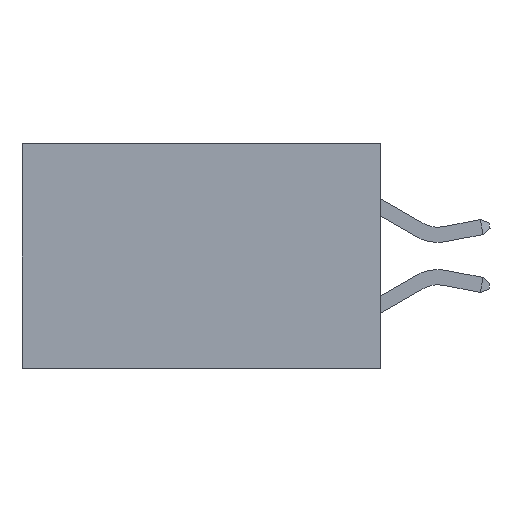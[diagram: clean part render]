
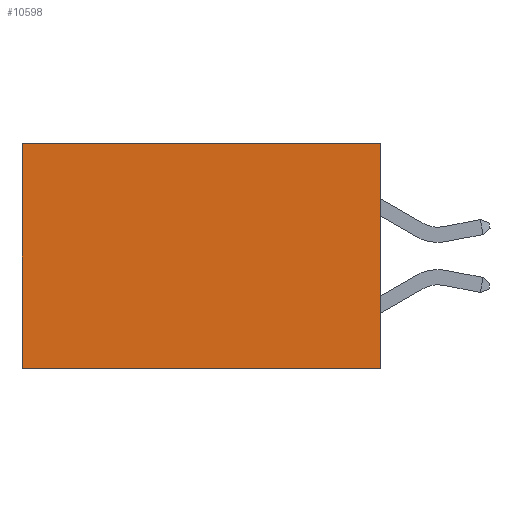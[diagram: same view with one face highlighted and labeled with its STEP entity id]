
A CAD part, left-side view. The second image highlights one B-rep face of the part: STEP entity #10598.
In plain terms, the highlighted planar face has unit normal (-1, 0, 0).
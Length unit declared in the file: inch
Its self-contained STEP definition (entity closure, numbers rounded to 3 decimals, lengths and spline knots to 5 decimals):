
#958 = CARTESIAN_POINT ( 'NONE',  ( 0.277, 0., -0.37 ) ) ;
#1121 = ORIENTED_EDGE ( 'NONE', *, *, #18309, .T. ) ;
#1343 = VECTOR ( 'NONE', #18178, 39.37008 ) ;
#1370 = EDGE_CURVE ( 'NONE', #19602, #3706, #2652, .T. ) ;
#2280 = VECTOR ( 'NONE', #15976, 39.37008 ) ;
#2432 = CARTESIAN_POINT ( 'NONE',  ( 0.277, 0.59, -0.37 ) ) ;
#2652 = LINE ( 'NONE', #958, #10940 ) ;
#3392 = VECTOR ( 'NONE', #19661, 39.37008 ) ;
#3411 = ORIENTED_EDGE ( 'NONE', *, *, #11830, .T. ) ;
#3706 = VERTEX_POINT ( 'NONE', #2432 ) ;
#3864 = CARTESIAN_POINT ( 'NONE',  ( 0.277, 0., 0. ) ) ;
#5876 = EDGE_CURVE ( 'NONE', #8529, #19602, #15855, .T. ) ;
#5952 = DIRECTION ( 'NONE',  ( 0., 1., 0. ) ) ;
#6285 = ORIENTED_EDGE ( 'NONE', *, *, #5876, .F. ) ;
#6649 = CARTESIAN_POINT ( 'NONE',  ( 0.277, 0.59, -0.37 ) ) ;
#6843 = FACE_OUTER_BOUND ( 'NONE', #8257, .T. ) ;
#8063 = VERTEX_POINT ( 'NONE', #20841 ) ;
#8257 = EDGE_LOOP ( 'NONE', ( #3411, #17084, #6285, #1121 ) ) ;
#8529 = VERTEX_POINT ( 'NONE', #3864 ) ;
#10288 = DIRECTION ( 'NONE',  ( 0., 0., -1. ) ) ;
#10598 = ADVANCED_FACE ( 'NONE', ( #6843 ), #10864, .F. ) ;
#10864 = PLANE ( 'NONE',  #12061 ) ;
#10940 = VECTOR ( 'NONE', #5952, 39.37008 ) ;
#11830 = EDGE_CURVE ( 'NONE', #8063, #3706, #16415, .T. ) ;
#12061 = AXIS2_PLACEMENT_3D ( 'NONE', #17284, #19988, #10288 ) ;
#13338 = CARTESIAN_POINT ( 'NONE',  ( 0.277, 0., 0. ) ) ;
#13960 = LINE ( 'NONE', #13338, #1343 ) ;
#15855 = LINE ( 'NONE', #15955, #2280 ) ;
#15955 = CARTESIAN_POINT ( 'NONE',  ( 0.277, 0., -0.37 ) ) ;
#15976 = DIRECTION ( 'NONE',  ( 0., 0., -1. ) ) ;
#16415 = LINE ( 'NONE', #6649, #3392 ) ;
#16774 = CARTESIAN_POINT ( 'NONE',  ( 0.277, 0., -0.37 ) ) ;
#17084 = ORIENTED_EDGE ( 'NONE', *, *, #1370, .F. ) ;
#17284 = CARTESIAN_POINT ( 'NONE',  ( 0.277, 0., -0.37 ) ) ;
#18178 = DIRECTION ( 'NONE',  ( 0., 1., 0. ) ) ;
#18309 = EDGE_CURVE ( 'NONE', #8529, #8063, #13960, .T. ) ;
#19602 = VERTEX_POINT ( 'NONE', #16774 ) ;
#19661 = DIRECTION ( 'NONE',  ( 0., 0., -1. ) ) ;
#19988 = DIRECTION ( 'NONE',  ( 1., 0., 0. ) ) ;
#20841 = CARTESIAN_POINT ( 'NONE',  ( 0.277, 0.59, 0. ) ) ;
